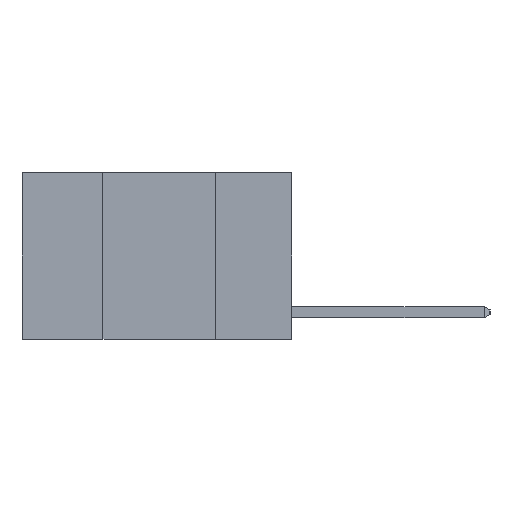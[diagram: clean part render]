
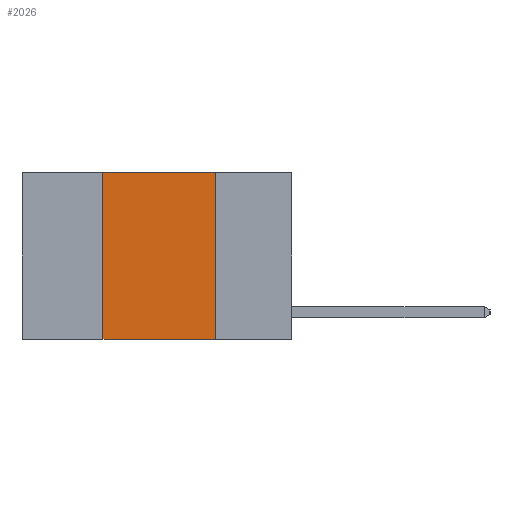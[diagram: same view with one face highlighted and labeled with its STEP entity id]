
A CAD part, left-side view. The second image highlights one B-rep face of the part: STEP entity #2026.
In plain terms, the highlighted planar face has unit normal (-1, 0, 0).
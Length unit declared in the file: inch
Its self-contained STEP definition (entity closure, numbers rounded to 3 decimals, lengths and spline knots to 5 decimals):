
#97 = CARTESIAN_POINT ( 'NONE',  ( 0., 0.6, -0.37 ) ) ;
#443 = FACE_OUTER_BOUND ( 'NONE', #6274, .T. ) ;
#1127 = CARTESIAN_POINT ( 'NONE',  ( 0., 0.42, -0.37 ) ) ;
#1404 = LINE ( 'NONE', #3221, #8351 ) ;
#1917 = EDGE_CURVE ( 'NONE', #7743, #4844, #3088, .T. ) ;
#2026 = ADVANCED_FACE ( 'NONE', ( #443 ), #7370, .F. ) ;
#2255 = CARTESIAN_POINT ( 'NONE',  ( 0., 0.17, -0.37 ) ) ;
#2756 = ORIENTED_EDGE ( 'NONE', *, *, #6331, .F. ) ;
#2772 = ORIENTED_EDGE ( 'NONE', *, *, #2867, .F. ) ;
#2867 = EDGE_CURVE ( 'NONE', #7743, #3411, #5108, .T. ) ;
#3088 = LINE ( 'NONE', #97, #6676 ) ;
#3094 = EDGE_CURVE ( 'NONE', #3411, #6694, #6146, .T. ) ;
#3221 = CARTESIAN_POINT ( 'NONE',  ( 0., 0.17, 0. ) ) ;
#3411 = VERTEX_POINT ( 'NONE', #4507 ) ;
#3591 = ORIENTED_EDGE ( 'NONE', *, *, #3094, .F. ) ;
#4507 = CARTESIAN_POINT ( 'NONE',  ( 0., 0.42, 0. ) ) ;
#4720 = DIRECTION ( 'NONE',  ( 0., 0., 1. ) ) ;
#4814 = CARTESIAN_POINT ( 'NONE',  ( 0., 0.42, 0. ) ) ;
#4844 = VERTEX_POINT ( 'NONE', #2255 ) ;
#5004 = DIRECTION ( 'NONE',  ( 0., -1., 0. ) ) ;
#5108 = LINE ( 'NONE', #4814, #8205 ) ;
#5129 = ORIENTED_EDGE ( 'NONE', *, *, #1917, .T. ) ;
#5676 = DIRECTION ( 'NONE',  ( 0., 0., -1. ) ) ;
#5898 = AXIS2_PLACEMENT_3D ( 'NONE', #8520, #7593, #5676 ) ;
#5936 = VECTOR ( 'NONE', #8656, 39.37008 ) ;
#5937 = DIRECTION ( 'NONE',  ( 0., 0., -1. ) ) ;
#5994 = CARTESIAN_POINT ( 'NONE',  ( 0., 0.6, 0. ) ) ;
#6146 = LINE ( 'NONE', #5994, #5936 ) ;
#6274 = EDGE_LOOP ( 'NONE', ( #2756, #3591, #2772, #5129 ) ) ;
#6331 = EDGE_CURVE ( 'NONE', #6694, #4844, #1404, .T. ) ;
#6676 = VECTOR ( 'NONE', #5004, 39.37008 ) ;
#6694 = VERTEX_POINT ( 'NONE', #7590 ) ;
#7370 = PLANE ( 'NONE',  #5898 ) ;
#7590 = CARTESIAN_POINT ( 'NONE',  ( 0., 0.17, 0. ) ) ;
#7593 = DIRECTION ( 'NONE',  ( 1., 0., 0. ) ) ;
#7743 = VERTEX_POINT ( 'NONE', #1127 ) ;
#8205 = VECTOR ( 'NONE', #4720, 39.37008 ) ;
#8351 = VECTOR ( 'NONE', #5937, 39.37008 ) ;
#8520 = CARTESIAN_POINT ( 'NONE',  ( 0., 0.6, 0. ) ) ;
#8656 = DIRECTION ( 'NONE',  ( 0., -1., 0. ) ) ;
